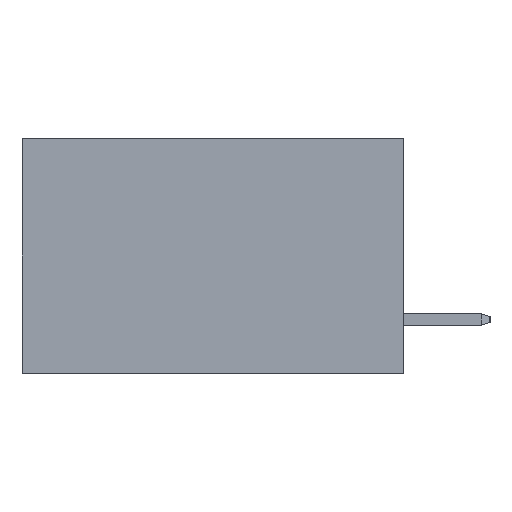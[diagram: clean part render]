
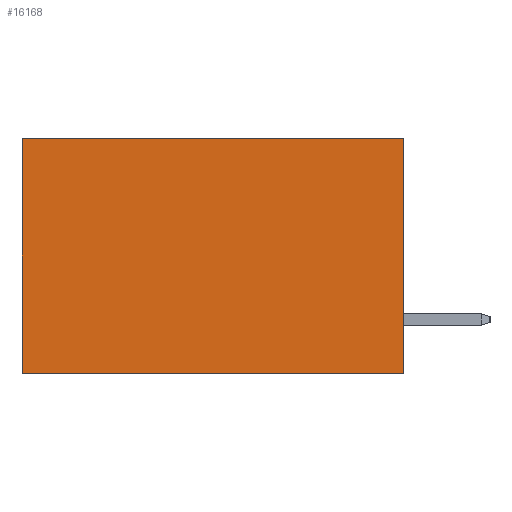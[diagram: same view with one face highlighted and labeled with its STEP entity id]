
A CAD part, left-side view. The second image highlights one B-rep face of the part: STEP entity #16168.
In plain terms, the highlighted planar face has unit normal (-1, 0, 0).
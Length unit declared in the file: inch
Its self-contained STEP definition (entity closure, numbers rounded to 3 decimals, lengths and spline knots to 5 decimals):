
#963 = CARTESIAN_POINT ( 'NONE',  ( 0.2875, 0.6, -0.37 ) ) ;
#1079 = DIRECTION ( 'NONE',  ( 0., 0., -1. ) ) ;
#1633 = VECTOR ( 'NONE', #7490, 39.37008 ) ;
#1735 = CARTESIAN_POINT ( 'NONE',  ( 0.2875, 0., 0. ) ) ;
#1996 = EDGE_CURVE ( 'NONE', #15425, #11646, #9583, .T. ) ;
#2295 = CARTESIAN_POINT ( 'NONE',  ( 0.2875, 0., -0.37 ) ) ;
#2324 = LINE ( 'NONE', #7441, #3388 ) ;
#3012 = EDGE_CURVE ( 'NONE', #11646, #6974, #8673, .T. ) ;
#3198 = CARTESIAN_POINT ( 'NONE',  ( 0.2875, 0., 0. ) ) ;
#3388 = VECTOR ( 'NONE', #1079, 39.37008 ) ;
#3797 = PLANE ( 'NONE',  #11259 ) ;
#3981 = VERTEX_POINT ( 'NONE', #11797 ) ;
#5049 = DIRECTION ( 'NONE',  ( 1., 0., 0. ) ) ;
#5085 = DIRECTION ( 'NONE',  ( 0., 1., 0. ) ) ;
#6357 = EDGE_CURVE ( 'NONE', #15425, #3981, #6426, .T. ) ;
#6426 = LINE ( 'NONE', #11546, #12614 ) ;
#6974 = VERTEX_POINT ( 'NONE', #963 ) ;
#7441 = CARTESIAN_POINT ( 'NONE',  ( 0.2875, 0.6, 0. ) ) ;
#7490 = DIRECTION ( 'NONE',  ( 0., 1., 0. ) ) ;
#7674 = ORIENTED_EDGE ( 'NONE', *, *, #1996, .F. ) ;
#8673 = LINE ( 'NONE', #2295, #1633 ) ;
#9369 = ORIENTED_EDGE ( 'NONE', *, *, #3012, .F. ) ;
#9583 = LINE ( 'NONE', #3198, #13339 ) ;
#11019 = EDGE_CURVE ( 'NONE', #3981, #6974, #2324, .T. ) ;
#11259 = AXIS2_PLACEMENT_3D ( 'NONE', #16563, #5049, #15380 ) ;
#11429 = FACE_OUTER_BOUND ( 'NONE', #15468, .T. ) ;
#11546 = CARTESIAN_POINT ( 'NONE',  ( 0.2875, 0., 0. ) ) ;
#11646 = VERTEX_POINT ( 'NONE', #13676 ) ;
#11797 = CARTESIAN_POINT ( 'NONE',  ( 0.2875, 0.6, 0. ) ) ;
#12085 = ORIENTED_EDGE ( 'NONE', *, *, #6357, .T. ) ;
#12322 = ORIENTED_EDGE ( 'NONE', *, *, #11019, .T. ) ;
#12614 = VECTOR ( 'NONE', #5085, 39.37008 ) ;
#13339 = VECTOR ( 'NONE', #13522, 39.37008 ) ;
#13522 = DIRECTION ( 'NONE',  ( 0., 0., -1. ) ) ;
#13676 = CARTESIAN_POINT ( 'NONE',  ( 0.2875, 0., -0.37 ) ) ;
#15380 = DIRECTION ( 'NONE',  ( 0., 0., -1. ) ) ;
#15425 = VERTEX_POINT ( 'NONE', #1735 ) ;
#15468 = EDGE_LOOP ( 'NONE', ( #12322, #9369, #7674, #12085 ) ) ;
#16168 = ADVANCED_FACE ( 'NONE', ( #11429 ), #3797, .F. ) ;
#16563 = CARTESIAN_POINT ( 'NONE',  ( 0.2875, 0., 0. ) ) ;
